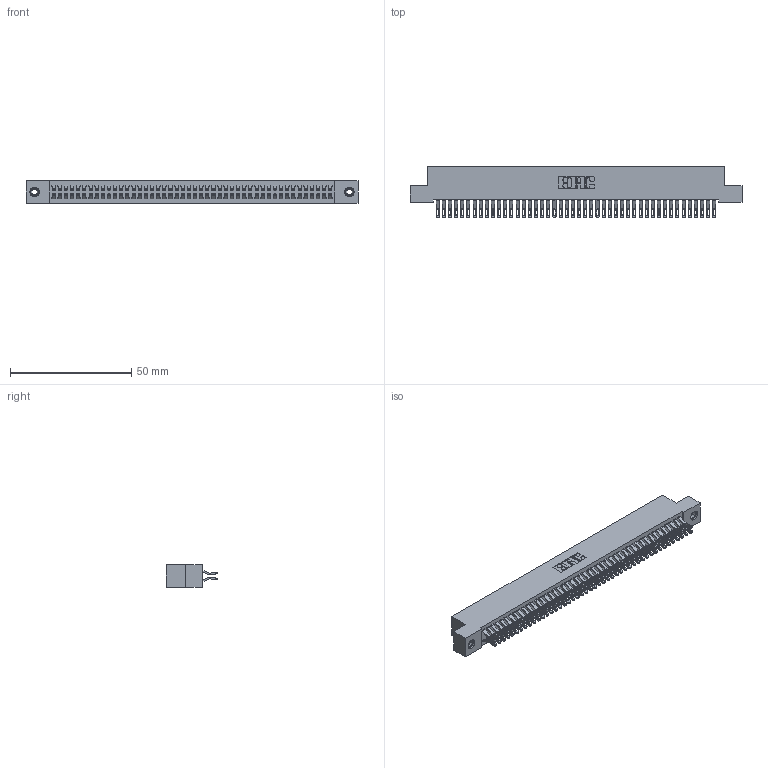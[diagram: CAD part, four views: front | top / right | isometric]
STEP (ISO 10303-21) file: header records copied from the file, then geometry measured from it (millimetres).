
FILE_DESCRIPTION (( 'STEP AP203' ), '1' );
FILE_NAME ('392-092-555-208.STEP', '2018-08-18T08:13:18', ( '' ), ( '' ), 'SwSTEP 2.0', 'SolidWorks 2016', '' );
FILE_SCHEMA (( 'CONFIG_CONTROL_DESIGN' ));
Length unit declared in the file: inch
Products named in the file (4): 342 Part_TI; 345-292-001_555 Tail; 345-250-001_345-250-003-102; 392-092-555-208
Assembly tree (95 placements, depth 2):
  392-092-555-208
    342 Part_TI
    345-292-001_555 Tail  x92
    345-250-001_345-250-003-102  x2
Bounding box: 137.16 x 21.47 x 9.4 mm (x, y, z)
Volume: 12592.7 mm3; surface area: 21496.8 mm2
Topology: 95 solids, 95 shells, 5506 faces, 17271 edges, 11506 vertices
Faces by surface type: plane 3226, cylinder 2264, cone 12, torus 4
Entity records: 30456 total; most frequent: CARTESIAN_POINT 5059, ORIENTED_EDGE 4958, DIRECTION 4317, EDGE_CURVE 2479, LINE 2311, VECTOR 2311, VERTEX_POINT 1648, AXIS2_PLACEMENT_3D 1003
